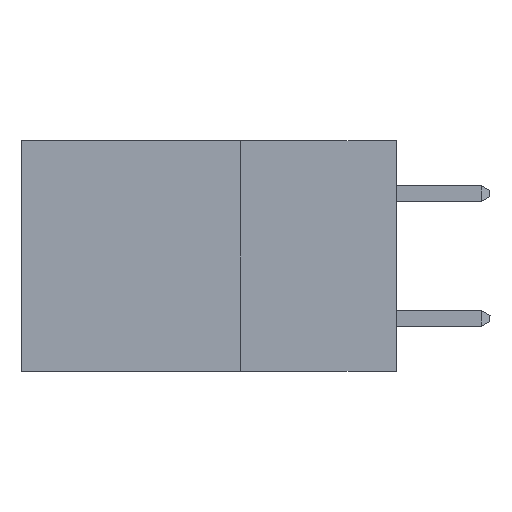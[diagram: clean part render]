
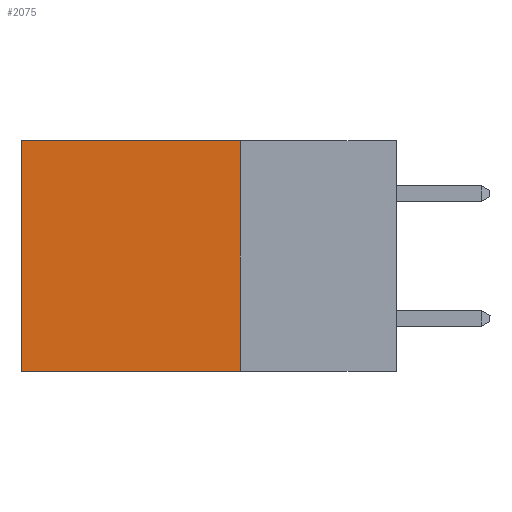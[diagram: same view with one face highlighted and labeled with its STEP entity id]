
A CAD part, left-side view. The second image highlights one B-rep face of the part: STEP entity #2075.
In plain terms, the highlighted planar face has unit normal (-1, 0, 0).
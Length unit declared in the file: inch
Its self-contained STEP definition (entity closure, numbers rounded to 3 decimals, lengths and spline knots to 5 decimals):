
#38 = VERTEX_POINT ( 'NONE', #3320 ) ;
#121 = ORIENTED_EDGE ( 'NONE', *, *, #2948, .F. ) ;
#239 = DIRECTION ( 'NONE',  ( 0., 1., 0. ) ) ;
#319 = CARTESIAN_POINT ( 'NONE',  ( 0.2615, 0.25, -0.37 ) ) ;
#420 = LINE ( 'NONE', #16875, #7484 ) ;
#865 = AXIS2_PLACEMENT_3D ( 'NONE', #10440, #15071, #16264 ) ;
#1155 = EDGE_LOOP ( 'NONE', ( #10065, #121, #2773, #10389 ) ) ;
#2075 = ADVANCED_FACE ( 'NONE', ( #9238 ), #14383, .F. ) ;
#2773 = ORIENTED_EDGE ( 'NONE', *, *, #16277, .F. ) ;
#2948 = EDGE_CURVE ( 'NONE', #10489, #38, #7042, .T. ) ;
#3188 = LINE ( 'NONE', #3620, #17721 ) ;
#3320 = CARTESIAN_POINT ( 'NONE',  ( 0.2615, 0.6, -0.37 ) ) ;
#3620 = CARTESIAN_POINT ( 'NONE',  ( 0.2615, 0.25, -0.37 ) ) ;
#3754 = VECTOR ( 'NONE', #239, 39.37008 ) ;
#5076 = CARTESIAN_POINT ( 'NONE',  ( 0.2615, 0.25, 0. ) ) ;
#5991 = DIRECTION ( 'NONE',  ( 0., 0., -1. ) ) ;
#6268 = EDGE_CURVE ( 'NONE', #11095, #12635, #17328, .T. ) ;
#7042 = LINE ( 'NONE', #319, #3754 ) ;
#7484 = VECTOR ( 'NONE', #5991, 39.37008 ) ;
#9238 = FACE_OUTER_BOUND ( 'NONE', #1155, .T. ) ;
#10065 = ORIENTED_EDGE ( 'NONE', *, *, #12538, .T. ) ;
#10389 = ORIENTED_EDGE ( 'NONE', *, *, #6268, .T. ) ;
#10440 = CARTESIAN_POINT ( 'NONE',  ( 0.2615, 0.25, -0.37 ) ) ;
#10489 = VERTEX_POINT ( 'NONE', #14042 ) ;
#11095 = VERTEX_POINT ( 'NONE', #16585 ) ;
#12538 = EDGE_CURVE ( 'NONE', #12635, #38, #420, .T. ) ;
#12635 = VERTEX_POINT ( 'NONE', #14375 ) ;
#13257 = DIRECTION ( 'NONE',  ( 0., 0., -1. ) ) ;
#14042 = CARTESIAN_POINT ( 'NONE',  ( 0.2615, 0.25, -0.37 ) ) ;
#14375 = CARTESIAN_POINT ( 'NONE',  ( 0.2615, 0.6, 0. ) ) ;
#14383 = PLANE ( 'NONE',  #865 ) ;
#15071 = DIRECTION ( 'NONE',  ( 1., 0., 0. ) ) ;
#16264 = DIRECTION ( 'NONE',  ( 0., 0., -1. ) ) ;
#16277 = EDGE_CURVE ( 'NONE', #11095, #10489, #3188, .T. ) ;
#16585 = CARTESIAN_POINT ( 'NONE',  ( 0.2615, 0.25, 0. ) ) ;
#16812 = DIRECTION ( 'NONE',  ( 0., 1., 0. ) ) ;
#16875 = CARTESIAN_POINT ( 'NONE',  ( 0.2615, 0.6, -0.37 ) ) ;
#16908 = VECTOR ( 'NONE', #16812, 39.37008 ) ;
#17328 = LINE ( 'NONE', #5076, #16908 ) ;
#17721 = VECTOR ( 'NONE', #13257, 39.37008 ) ;
